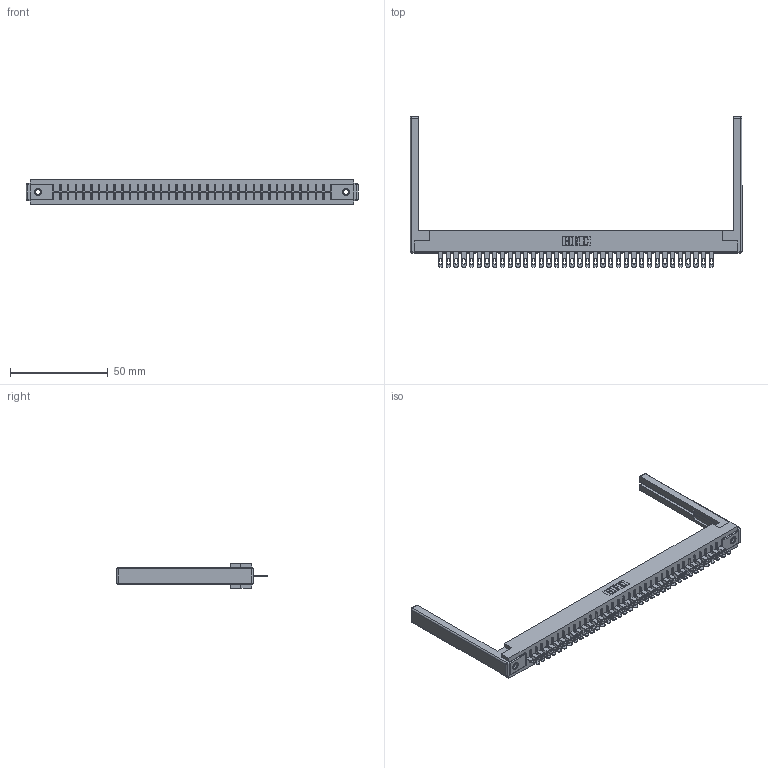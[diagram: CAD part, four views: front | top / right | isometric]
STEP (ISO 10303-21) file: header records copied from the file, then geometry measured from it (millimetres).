
FILE_DESCRIPTION (( 'STEP AP203' ), '1' );
FILE_NAME ('316-036-400-168.STEP', '2020-09-23T04:58:29', ( '' ), ( '' ), 'SwSTEP 2.0', 'SolidWorks 2020', '' );
FILE_SCHEMA (( 'CONFIG_CONTROL_DESIGN' ));
Length unit declared in the file: inch
Products named in the file (5): 307-220-068; 306 Part_.156 Dia; 316-036-400-168; 345-250-001_345-250-001-102; 306-290-001_100
Assembly tree (41 placements, depth 2):
  316-036-400-168
    306 Part_.156 Dia
    306-290-001_100  x36
    345-250-001_345-250-001-102  x2
    307-220-068  x2
Bounding box: 170.08 x 77.17 x 12.7 mm (x, y, z)
Volume: 23238.3 mm3; surface area: 23991.8 mm2
Topology: 41 solids, 41 shells, 3006 faces, 8446 edges, 5416 vertices
Faces by surface type: plane 1956, cylinder 882, sphere 152, cone 12, torus 4
Entity records: 37272 total; most frequent: CARTESIAN_POINT 6224, ORIENTED_EDGE 6162, DIRECTION 6151, EDGE_CURVE 3081, VECTOR 2401, LINE 2401, VERTEX_POINT 1948, AXIS2_PLACEMENT_3D 1875
